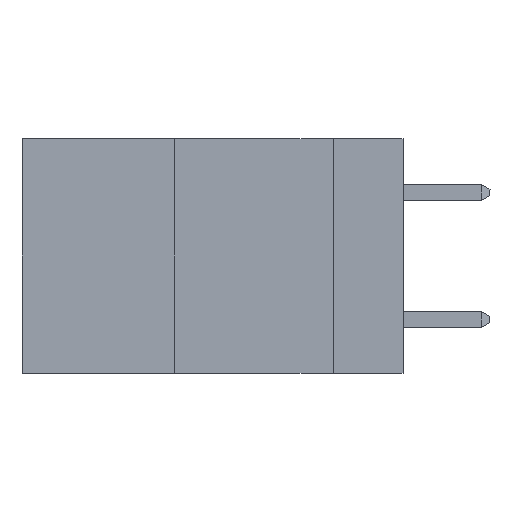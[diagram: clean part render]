
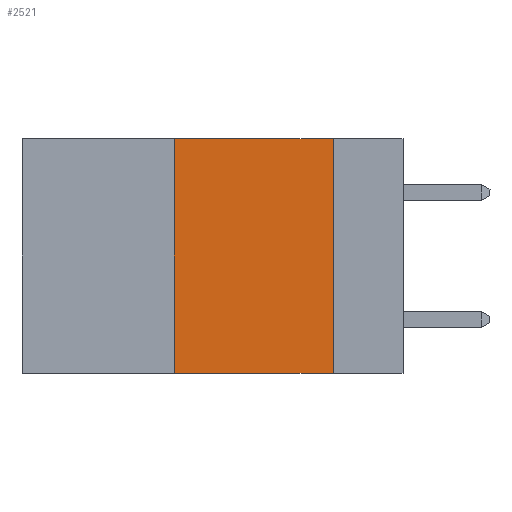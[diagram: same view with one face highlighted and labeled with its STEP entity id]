
A CAD part, left-side view. The second image highlights one B-rep face of the part: STEP entity #2521.
In plain terms, the highlighted planar face has unit normal (-1, 0, 0).
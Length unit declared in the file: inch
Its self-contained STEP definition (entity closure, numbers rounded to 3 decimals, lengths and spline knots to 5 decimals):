
#341 = LINE ( 'NONE', #9431, #1044 ) ;
#418 = VERTEX_POINT ( 'NONE', #6407 ) ;
#466 = LINE ( 'NONE', #6571, #5789 ) ;
#526 = ORIENTED_EDGE ( 'NONE', *, *, #1336, .F. ) ;
#1044 = VECTOR ( 'NONE', #6378, 39.37008 ) ;
#1216 = VERTEX_POINT ( 'NONE', #5451 ) ;
#1336 = EDGE_CURVE ( 'NONE', #1216, #418, #2279, .T. ) ;
#1360 = VERTEX_POINT ( 'NONE', #9628 ) ;
#1813 = CARTESIAN_POINT ( 'NONE',  ( 0., 0.11, 0. ) ) ;
#2086 = ORIENTED_EDGE ( 'NONE', *, *, #3017, .F. ) ;
#2279 = LINE ( 'NONE', #1813, #4392 ) ;
#2389 = LINE ( 'NONE', #9230, #8245 ) ;
#2521 = ADVANCED_FACE ( 'NONE', ( #8798 ), #7571, .F. ) ;
#2637 = DIRECTION ( 'NONE',  ( 0., 0., -1. ) ) ;
#2897 = EDGE_LOOP ( 'NONE', ( #526, #5214, #2086, #9716 ) ) ;
#3016 = CARTESIAN_POINT ( 'NONE',  ( 0., 0.6, 0. ) ) ;
#3017 = EDGE_CURVE ( 'NONE', #1360, #8371, #341, .T. ) ;
#3044 = DIRECTION ( 'NONE',  ( 0., 0., -1. ) ) ;
#3053 = AXIS2_PLACEMENT_3D ( 'NONE', #3016, #9066, #3044 ) ;
#4329 = DIRECTION ( 'NONE',  ( 0., -1., 0. ) ) ;
#4392 = VECTOR ( 'NONE', #2637, 39.37008 ) ;
#5214 = ORIENTED_EDGE ( 'NONE', *, *, #9675, .F. ) ;
#5451 = CARTESIAN_POINT ( 'NONE',  ( 0., 0.11, 0. ) ) ;
#5789 = VECTOR ( 'NONE', #7505, 39.37008 ) ;
#6378 = DIRECTION ( 'NONE',  ( 0., 0., 1. ) ) ;
#6407 = CARTESIAN_POINT ( 'NONE',  ( 0., 0.11, -0.37 ) ) ;
#6571 = CARTESIAN_POINT ( 'NONE',  ( 0., 0.6, 0. ) ) ;
#7505 = DIRECTION ( 'NONE',  ( 0., -1., 0. ) ) ;
#7571 = PLANE ( 'NONE',  #3053 ) ;
#8245 = VECTOR ( 'NONE', #4329, 39.37008 ) ;
#8371 = VERTEX_POINT ( 'NONE', #8982 ) ;
#8798 = FACE_OUTER_BOUND ( 'NONE', #2897, .T. ) ;
#8932 = EDGE_CURVE ( 'NONE', #1360, #418, #2389, .T. ) ;
#8982 = CARTESIAN_POINT ( 'NONE',  ( 0., 0.36, 0. ) ) ;
#9066 = DIRECTION ( 'NONE',  ( 1., 0., 0. ) ) ;
#9230 = CARTESIAN_POINT ( 'NONE',  ( 0., 0.6, -0.37 ) ) ;
#9431 = CARTESIAN_POINT ( 'NONE',  ( 0., 0.36, 0. ) ) ;
#9628 = CARTESIAN_POINT ( 'NONE',  ( 0., 0.36, -0.37 ) ) ;
#9675 = EDGE_CURVE ( 'NONE', #8371, #1216, #466, .T. ) ;
#9716 = ORIENTED_EDGE ( 'NONE', *, *, #8932, .T. ) ;
